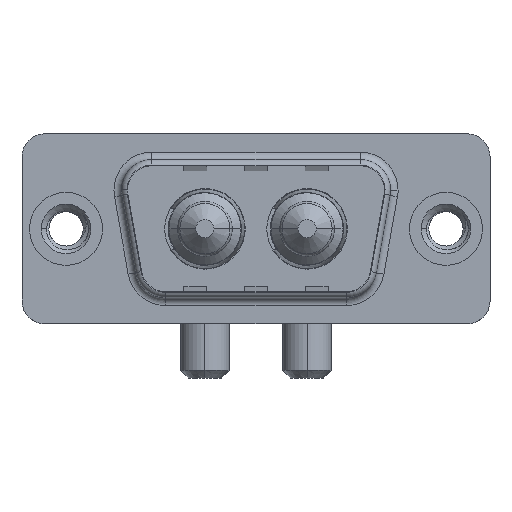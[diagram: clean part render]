
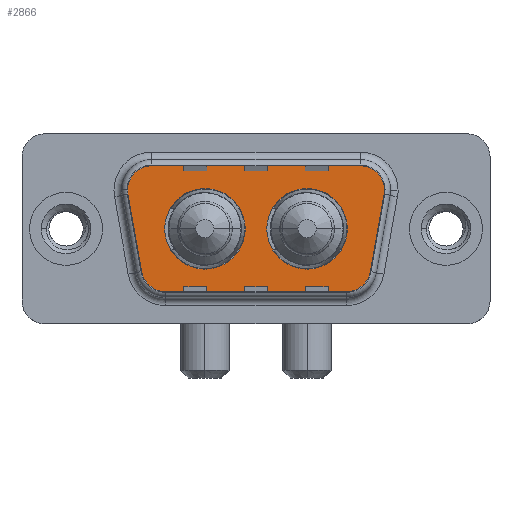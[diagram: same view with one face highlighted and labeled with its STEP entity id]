
A CAD part, top view. The second image highlights one B-rep face of the part: STEP entity #2866.
In plain terms, the highlighted planar face has unit normal (0, 0, 1).
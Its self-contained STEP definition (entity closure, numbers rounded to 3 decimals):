
#39 = VERTEX_POINT ( 'NONE', #2524 ) ;
#184 = DIRECTION ( 'NONE',  ( 0., 0., 1. ) ) ;
#316 = AXIS2_PLACEMENT_3D ( 'NONE', #5421, #184, #9903 ) ;
#580 = CARTESIAN_POINT ( 'NONE',  ( 18.51, 0., 0. ) ) ;
#846 = CARTESIAN_POINT ( 'NONE',  ( 3.466, 2.553, 0. ) ) ;
#1029 = CARTESIAN_POINT ( 'NONE',  ( 6.459, -2.9, 0. ) ) ;
#1071 = VERTEX_POINT ( 'NONE', #10497 ) ;
#1095 = VERTEX_POINT ( 'NONE', #2479 ) ;
#1097 = VECTOR ( 'NONE', #1403, 1000. ) ;
#1310 = CARTESIAN_POINT ( 'NONE',  ( 11.79, 0., 0. ) ) ;
#1393 = EDGE_CURVE ( 'NONE', #39, #10367, #1492, .T. ) ;
#1403 = DIRECTION ( 'NONE',  ( 0.174, 0.985, 0. ) ) ;
#1492 = CIRCLE ( 'NONE', #5254, 2.65 ) ;
#1498 = DIRECTION ( 'NONE',  ( 0., 0., 1. ) ) ;
#1642 = LINE ( 'NONE', #11322, #1097 ) ;
#1764 = FACE_BOUND ( 'NONE', #7174, .T. ) ;
#1767 = CARTESIAN_POINT ( 'NONE',  ( 5.436, 4.9, 0. ) ) ;
#1911 = EDGE_CURVE ( 'NONE', #11158, #1095, #5295, .T. ) ;
#1967 = DIRECTION ( 'NONE',  ( -1., 0., 0. ) ) ;
#2136 = ORIENTED_EDGE ( 'NONE', *, *, #2720, .T. ) ;
#2158 = ORIENTED_EDGE ( 'NONE', *, *, #11374, .T. ) ;
#2479 = CARTESIAN_POINT ( 'NONE',  ( 6.459, -4.9, 0. ) ) ;
#2511 = DIRECTION ( 'NONE',  ( 1., 0., 0. ) ) ;
#2524 = CARTESIAN_POINT ( 'NONE',  ( 6.49, 0., 0. ) ) ;
#2586 = LINE ( 'NONE', #11552, #3539 ) ;
#2720 = EDGE_CURVE ( 'NONE', #10852, #7133, #8259, .T. ) ;
#2761 = DIRECTION ( 'NONE',  ( 0., 0., 1. ) ) ;
#2838 = EDGE_CURVE ( 'NONE', #9537, #11158, #4580, .T. ) ;
#2866 = ADVANCED_FACE ( 'NONE', ( #1764, #9832, #11496 ), #7216, .T. ) ;
#3000 = CARTESIAN_POINT ( 'NONE',  ( 20.511, -3.247, 0. ) ) ;
#3100 = VECTOR ( 'NONE', #4810, 1000. ) ;
#3234 = DIRECTION ( 'NONE',  ( 1., 0., 0. ) ) ;
#3239 = DIRECTION ( 'NONE',  ( 0., 0., 1. ) ) ;
#3293 = ORIENTED_EDGE ( 'NONE', *, *, #6458, .T. ) ;
#3431 = AXIS2_PLACEMENT_3D ( 'NONE', #4285, #10477, #3234 ) ;
#3539 = VECTOR ( 'NONE', #9719, 1000. ) ;
#3548 = VERTEX_POINT ( 'NONE', #4230 ) ;
#3697 = CARTESIAN_POINT ( 'NONE',  ( 3.466, 2.553, 0. ) ) ;
#3794 = AXIS2_PLACEMENT_3D ( 'NONE', #9429, #3239, #10484 ) ;
#3942 = ORIENTED_EDGE ( 'NONE', *, *, #1911, .T. ) ;
#3963 = VERTEX_POINT ( 'NONE', #580 ) ;
#4018 = EDGE_CURVE ( 'NONE', #10367, #39, #8836, .T. ) ;
#4230 = CARTESIAN_POINT ( 'NONE',  ( 21.534, 2.553, 0. ) ) ;
#4285 = CARTESIAN_POINT ( 'NONE',  ( 9.14, 0., 0. ) ) ;
#4310 = CIRCLE ( 'NONE', #10277, 2.65 ) ;
#4396 = DIRECTION ( 'NONE',  ( -1., 0., 0. ) ) ;
#4409 = CARTESIAN_POINT ( 'NONE',  ( 18.541, -2.9, 0. ) ) ;
#4448 = ORIENTED_EDGE ( 'NONE', *, *, #4018, .F. ) ;
#4580 = LINE ( 'NONE', #3697, #6764 ) ;
#4810 = DIRECTION ( 'NONE',  ( -1., 0., 0. ) ) ;
#5093 = DIRECTION ( 'NONE',  ( 0., 0., 1. ) ) ;
#5254 = AXIS2_PLACEMENT_3D ( 'NONE', #10546, #2761, #10599 ) ;
#5295 = CIRCLE ( 'NONE', #6782, 2. ) ;
#5421 = CARTESIAN_POINT ( 'NONE',  ( 5.436, 2.9, 0. ) ) ;
#5464 = AXIS2_PLACEMENT_3D ( 'NONE', #4409, #6218, #8780 ) ;
#5615 = AXIS2_PLACEMENT_3D ( 'NONE', #7021, #1498, #2511 ) ;
#5902 = ORIENTED_EDGE ( 'NONE', *, *, #6132, .T. ) ;
#5916 = CARTESIAN_POINT ( 'NONE',  ( 5.436, 4.9, 0. ) ) ;
#6087 = DIRECTION ( 'NONE',  ( 1., 0., 0. ) ) ;
#6132 = EDGE_CURVE ( 'NONE', #10799, #8692, #6854, .T. ) ;
#6202 = EDGE_LOOP ( 'NONE', ( #4448, #7626 ) ) ;
#6218 = DIRECTION ( 'NONE',  ( 0., 0., 1. ) ) ;
#6447 = ORIENTED_EDGE ( 'NONE', *, *, #8888, .F. ) ;
#6458 = EDGE_CURVE ( 'NONE', #8692, #9537, #10413, .T. ) ;
#6584 = CARTESIAN_POINT ( 'NONE',  ( 19.564, 4.9, 0. ) ) ;
#6764 = VECTOR ( 'NONE', #10662, 1000. ) ;
#6782 = AXIS2_PLACEMENT_3D ( 'NONE', #1029, #7301, #1967 ) ;
#6786 = VERTEX_POINT ( 'NONE', #10553 ) ;
#6854 = LINE ( 'NONE', #5916, #3100 ) ;
#6904 = CARTESIAN_POINT ( 'NONE',  ( 19.564, 2.9, 0. ) ) ;
#6911 = ORIENTED_EDGE ( 'NONE', *, *, #8640, .T. ) ;
#6919 = AXIS2_PLACEMENT_3D ( 'NONE', #10530, #7944, #10349 ) ;
#7002 = ORIENTED_EDGE ( 'NONE', *, *, #8999, .T. ) ;
#7021 = CARTESIAN_POINT ( 'NONE',  ( 15.86, 0., 0. ) ) ;
#7026 = DIRECTION ( 'NONE',  ( 0., 0., 1. ) ) ;
#7133 = VERTEX_POINT ( 'NONE', #3000 ) ;
#7174 = EDGE_LOOP ( 'NONE', ( #6447, #9303 ) ) ;
#7216 = PLANE ( 'NONE',  #5464 ) ;
#7301 = DIRECTION ( 'NONE',  ( 0., 0., 1. ) ) ;
#7626 = ORIENTED_EDGE ( 'NONE', *, *, #1393, .F. ) ;
#7944 = DIRECTION ( 'NONE',  ( 0., 0., 1. ) ) ;
#8025 = CIRCLE ( 'NONE', #5615, 2.65 ) ;
#8200 = EDGE_CURVE ( 'NONE', #7133, #3548, #1642, .T. ) ;
#8259 = CIRCLE ( 'NONE', #3794, 2. ) ;
#8531 = CARTESIAN_POINT ( 'NONE',  ( 4.489, -3.247, 0. ) ) ;
#8640 = EDGE_CURVE ( 'NONE', #1095, #10852, #2586, .T. ) ;
#8692 = VERTEX_POINT ( 'NONE', #1767 ) ;
#8778 = CIRCLE ( 'NONE', #6919, 2. ) ;
#8780 = DIRECTION ( 'NONE',  ( 1., 0., 0. ) ) ;
#8835 = AXIS2_PLACEMENT_3D ( 'NONE', #6904, #7026, #4396 ) ;
#8836 = CIRCLE ( 'NONE', #3431, 2.65 ) ;
#8888 = EDGE_CURVE ( 'NONE', #3963, #1071, #8025, .T. ) ;
#8904 = EDGE_CURVE ( 'NONE', #1071, #3963, #4310, .T. ) ;
#8999 = EDGE_CURVE ( 'NONE', #6786, #10799, #8778, .T. ) ;
#9302 = ORIENTED_EDGE ( 'NONE', *, *, #2838, .T. ) ;
#9303 = ORIENTED_EDGE ( 'NONE', *, *, #8904, .F. ) ;
#9429 = CARTESIAN_POINT ( 'NONE',  ( 18.541, -2.9, 0. ) ) ;
#9537 = VERTEX_POINT ( 'NONE', #846 ) ;
#9719 = DIRECTION ( 'NONE',  ( 1., 0., 0. ) ) ;
#9832 = FACE_BOUND ( 'NONE', #6202, .T. ) ;
#9903 = DIRECTION ( 'NONE',  ( 1., 0., 0. ) ) ;
#10083 = CARTESIAN_POINT ( 'NONE',  ( 18.541, -4.9, 0. ) ) ;
#10277 = AXIS2_PLACEMENT_3D ( 'NONE', #10585, #5093, #6087 ) ;
#10329 = CIRCLE ( 'NONE', #8835, 2. ) ;
#10349 = DIRECTION ( 'NONE',  ( -1., 0., 0. ) ) ;
#10367 = VERTEX_POINT ( 'NONE', #1310 ) ;
#10413 = CIRCLE ( 'NONE', #316, 2. ) ;
#10477 = DIRECTION ( 'NONE',  ( 0., 0., 1. ) ) ;
#10484 = DIRECTION ( 'NONE',  ( 1., 0., 0. ) ) ;
#10497 = CARTESIAN_POINT ( 'NONE',  ( 13.21, 0., 0. ) ) ;
#10530 = CARTESIAN_POINT ( 'NONE',  ( 19.564, 2.9, 0. ) ) ;
#10546 = CARTESIAN_POINT ( 'NONE',  ( 9.14, 0., 0. ) ) ;
#10553 = CARTESIAN_POINT ( 'NONE',  ( 21.564, 2.9, 0. ) ) ;
#10585 = CARTESIAN_POINT ( 'NONE',  ( 15.86, 0., 0. ) ) ;
#10599 = DIRECTION ( 'NONE',  ( 1., 0., 0. ) ) ;
#10630 = ORIENTED_EDGE ( 'NONE', *, *, #8200, .T. ) ;
#10662 = DIRECTION ( 'NONE',  ( 0.174, -0.985, 0. ) ) ;
#10799 = VERTEX_POINT ( 'NONE', #6584 ) ;
#10852 = VERTEX_POINT ( 'NONE', #10083 ) ;
#11158 = VERTEX_POINT ( 'NONE', #8531 ) ;
#11322 = CARTESIAN_POINT ( 'NONE',  ( 21.534, 2.553, 0. ) ) ;
#11374 = EDGE_CURVE ( 'NONE', #3548, #6786, #10329, .T. ) ;
#11395 = EDGE_LOOP ( 'NONE', ( #2136, #10630, #2158, #7002, #5902, #3293, #9302, #3942, #6911 ) ) ;
#11496 = FACE_OUTER_BOUND ( 'NONE', #11395, .T. ) ;
#11552 = CARTESIAN_POINT ( 'NONE',  ( 6.459, -4.9, 0. ) ) ;
